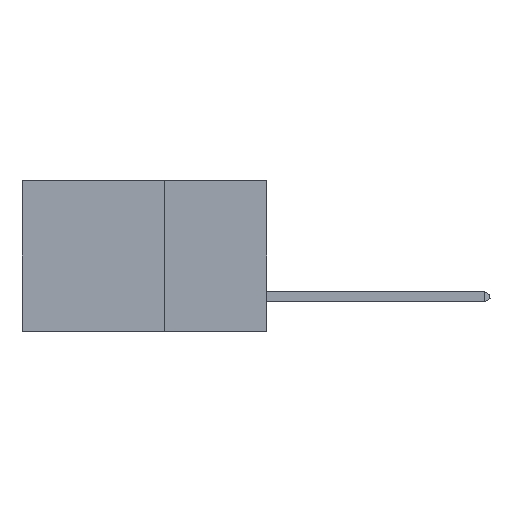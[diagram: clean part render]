
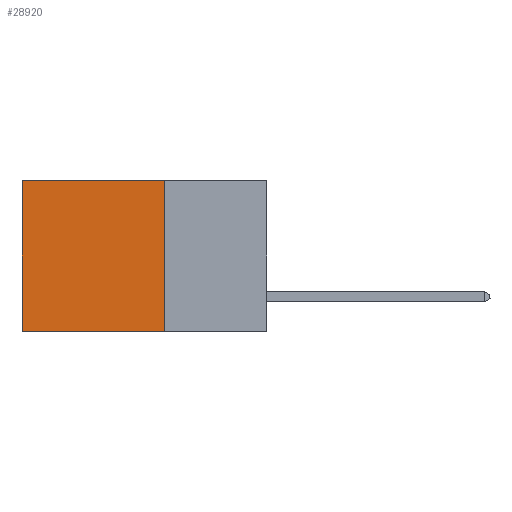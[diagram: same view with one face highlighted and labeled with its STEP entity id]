
A CAD part, left-side view. The second image highlights one B-rep face of the part: STEP entity #28920.
In plain terms, the highlighted planar face has unit normal (-1, 0, 0).
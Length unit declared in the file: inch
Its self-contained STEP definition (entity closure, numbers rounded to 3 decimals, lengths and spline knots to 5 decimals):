
#519 = CARTESIAN_POINT ( 'NONE',  ( 0.2875, 0.25, 0. ) ) ;
#640 = DIRECTION ( 'NONE',  ( 0., 0., -1. ) ) ;
#2490 = AXIS2_PLACEMENT_3D ( 'NONE', #17391, #9061, #28281 ) ;
#3468 = CARTESIAN_POINT ( 'NONE',  ( 0.2875, 0.6, 0. ) ) ;
#4555 = CARTESIAN_POINT ( 'NONE',  ( 0.2875, 0.6, 0. ) ) ;
#4564 = CARTESIAN_POINT ( 'NONE',  ( 0.2875, 0.25, -0.37 ) ) ;
#4648 = EDGE_CURVE ( 'NONE', #16223, #24099, #15327, .T. ) ;
#4986 = VECTOR ( 'NONE', #14784, 39.37008 ) ;
#6235 = VECTOR ( 'NONE', #11196, 39.37008 ) ;
#7671 = VERTEX_POINT ( 'NONE', #4564 ) ;
#8490 = ORIENTED_EDGE ( 'NONE', *, *, #16655, .F. ) ;
#9061 = DIRECTION ( 'NONE',  ( 1., 0., 0. ) ) ;
#11196 = DIRECTION ( 'NONE',  ( 0., 1., 0. ) ) ;
#14784 = DIRECTION ( 'NONE',  ( 0., 1., 0. ) ) ;
#15034 = ORIENTED_EDGE ( 'NONE', *, *, #29584, .T. ) ;
#15327 = LINE ( 'NONE', #3468, #35015 ) ;
#15574 = ORIENTED_EDGE ( 'NONE', *, *, #32820, .F. ) ;
#16223 = VERTEX_POINT ( 'NONE', #4555 ) ;
#16655 = EDGE_CURVE ( 'NONE', #33175, #7671, #34568, .T. ) ;
#17391 = CARTESIAN_POINT ( 'NONE',  ( 0.2875, 0.25, 0. ) ) ;
#17767 = ORIENTED_EDGE ( 'NONE', *, *, #4648, .T. ) ;
#20207 = CARTESIAN_POINT ( 'NONE',  ( 0.2875, 0.25, 0. ) ) ;
#20386 = VECTOR ( 'NONE', #640, 39.37008 ) ;
#20657 = DIRECTION ( 'NONE',  ( 0., 0., -1. ) ) ;
#21085 = CARTESIAN_POINT ( 'NONE',  ( 0.2875, 0.25, 0. ) ) ;
#22262 = CARTESIAN_POINT ( 'NONE',  ( 0.2875, 0.25, -0.37 ) ) ;
#23092 = CARTESIAN_POINT ( 'NONE',  ( 0.2875, 0.6, -0.37 ) ) ;
#24099 = VERTEX_POINT ( 'NONE', #23092 ) ;
#25559 = PLANE ( 'NONE',  #2490 ) ;
#28265 = EDGE_LOOP ( 'NONE', ( #17767, #15574, #8490, #15034 ) ) ;
#28281 = DIRECTION ( 'NONE',  ( 0., 0., -1. ) ) ;
#28920 = ADVANCED_FACE ( 'NONE', ( #33648 ), #25559, .F. ) ;
#29584 = EDGE_CURVE ( 'NONE', #33175, #16223, #34007, .T. ) ;
#32820 = EDGE_CURVE ( 'NONE', #7671, #24099, #33568, .T. ) ;
#33175 = VERTEX_POINT ( 'NONE', #21085 ) ;
#33568 = LINE ( 'NONE', #22262, #6235 ) ;
#33648 = FACE_OUTER_BOUND ( 'NONE', #28265, .T. ) ;
#34007 = LINE ( 'NONE', #20207, #4986 ) ;
#34568 = LINE ( 'NONE', #519, #20386 ) ;
#35015 = VECTOR ( 'NONE', #20657, 39.37008 ) ;
